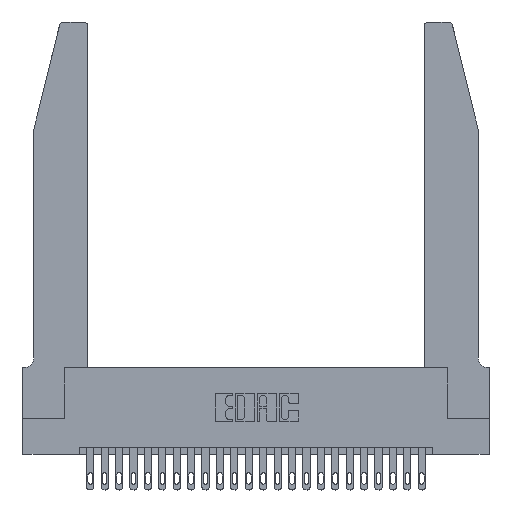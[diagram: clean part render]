
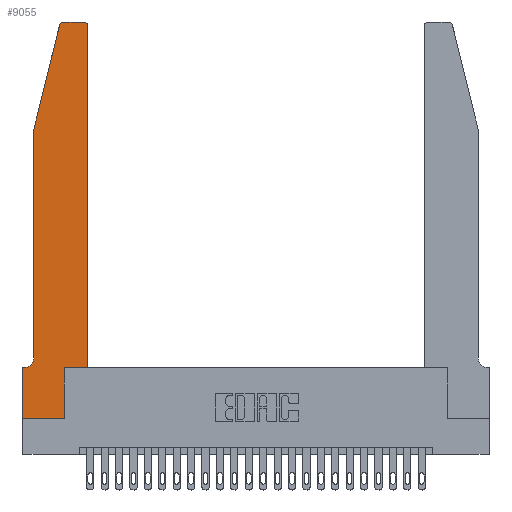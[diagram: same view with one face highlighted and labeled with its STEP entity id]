
A CAD part, top view. The second image highlights one B-rep face of the part: STEP entity #9055.
In plain terms, the highlighted planar face has unit normal (0, 0, 1).
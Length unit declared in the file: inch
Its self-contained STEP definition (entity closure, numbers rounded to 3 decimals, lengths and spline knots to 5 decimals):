
#1012 = VERTEX_POINT ( 'NONE', #17321 ) ;
#1343 = CARTESIAN_POINT ( 'NONE',  ( 0., 0., 0.37 ) ) ;
#1408 = DIRECTION ( 'NONE',  ( 0., 1., 0. ) ) ;
#1774 = ORIENTED_EDGE ( 'NONE', *, *, #21455, .T. ) ;
#2021 = VECTOR ( 'NONE', #23452, 39.37008 ) ;
#2440 = DIRECTION ( 'NONE',  ( -1., 0., 0. ) ) ;
#2599 = EDGE_CURVE ( 'NONE', #18158, #19687, #8711, .T. ) ;
#2645 = DIRECTION ( 'NONE',  ( 0., 0., 1. ) ) ;
#3170 = EDGE_CURVE ( 'NONE', #3212, #18158, #3987, .T. ) ;
#3212 = VERTEX_POINT ( 'NONE', #15938 ) ;
#3429 = LINE ( 'NONE', #4172, #18777 ) ;
#3468 = CARTESIAN_POINT ( 'NONE',  ( 0., 0., 0.37 ) ) ;
#3589 = LINE ( 'NONE', #13420, #18945 ) ;
#3613 = DIRECTION ( 'NONE',  ( 1., 0., 0. ) ) ;
#3987 = CIRCLE ( 'NONE', #25362, 0.03 ) ;
#4172 = CARTESIAN_POINT ( 'NONE',  ( 0.0755, 2., 0.37 ) ) ;
#4646 = VERTEX_POINT ( 'NONE', #13422 ) ;
#5094 = DIRECTION ( 'NONE',  ( 1., 0., 0. ) ) ;
#5379 = PLANE ( 'NONE',  #23579 ) ;
#6235 = CARTESIAN_POINT ( 'NONE',  ( 0.0755, 0.42, 0.37 ) ) ;
#7421 = EDGE_LOOP ( 'NONE', ( #23063, #25042, #14015, #12575, #7862, #16063, #1774, #9304, #20568, #23384, #13926, #14810 ) ) ;
#7805 = CARTESIAN_POINT ( 'NONE',  ( 0., 0.35, 0.37 ) ) ;
#7862 = ORIENTED_EDGE ( 'NONE', *, *, #20264, .T. ) ;
#8271 = CARTESIAN_POINT ( 'NONE',  ( 0.284, 2.75, 0.37 ) ) ;
#8536 = CARTESIAN_POINT ( 'NONE',  ( 0.284, 2.72, 0.37 ) ) ;
#8590 = CIRCLE ( 'NONE', #21376, 0.07 ) ;
#8711 = LINE ( 'NONE', #22270, #19089 ) ;
#8973 = VERTEX_POINT ( 'NONE', #1343 ) ;
#8981 = CARTESIAN_POINT ( 'NONE',  ( 0.2865, 0.35, 0.37 ) ) ;
#9055 = ADVANCED_FACE ( 'NONE', ( #25310 ), #5379, .T. ) ;
#9200 = LINE ( 'NONE', #11161, #15193 ) ;
#9304 = ORIENTED_EDGE ( 'NONE', *, *, #12291, .T. ) ;
#10670 = VECTOR ( 'NONE', #2440, 39.37008 ) ;
#11161 = CARTESIAN_POINT ( 'NONE',  ( 0., 0., 0.37 ) ) ;
#11275 = CIRCLE ( 'NONE', #17586, 0.03 ) ;
#11590 = VECTOR ( 'NONE', #5094, 39.37008 ) ;
#11944 = VERTEX_POINT ( 'NONE', #13131 ) ;
#12291 = EDGE_CURVE ( 'NONE', #8973, #13692, #16488, .T. ) ;
#12392 = DIRECTION ( 'NONE',  ( 1., 0., 0. ) ) ;
#12575 = ORIENTED_EDGE ( 'NONE', *, *, #21598, .T. ) ;
#13131 = CARTESIAN_POINT ( 'NONE',  ( 0.0755, 2., 0.37 ) ) ;
#13197 = CARTESIAN_POINT ( 'NONE',  ( 0.0055, 0.42, 0.37 ) ) ;
#13231 = VERTEX_POINT ( 'NONE', #8981 ) ;
#13420 = CARTESIAN_POINT ( 'NONE',  ( 0.0755, 2., 0.37 ) ) ;
#13422 = CARTESIAN_POINT ( 'NONE',  ( 0.0055, 0.35, 0.37 ) ) ;
#13692 = VERTEX_POINT ( 'NONE', #22928 ) ;
#13926 = ORIENTED_EDGE ( 'NONE', *, *, #18856, .T. ) ;
#14015 = ORIENTED_EDGE ( 'NONE', *, *, #17747, .T. ) ;
#14810 = ORIENTED_EDGE ( 'NONE', *, *, #3170, .T. ) ;
#15193 = VECTOR ( 'NONE', #19287, 39.37008 ) ;
#15235 = VECTOR ( 'NONE', #19707, 39.37008 ) ;
#15590 = LINE ( 'NONE', #16941, #23120 ) ;
#15938 = CARTESIAN_POINT ( 'NONE',  ( 0.4505, 2.72, 0.37 ) ) ;
#16063 = ORIENTED_EDGE ( 'NONE', *, *, #25273, .T. ) ;
#16488 = LINE ( 'NONE', #3468, #15235 ) ;
#16679 = VERTEX_POINT ( 'NONE', #6235 ) ;
#16941 = CARTESIAN_POINT ( 'NONE',  ( 0.4505, 0.35, 0.37 ) ) ;
#17083 = CARTESIAN_POINT ( 'NONE',  ( 0.4505, 0.35, 0.37 ) ) ;
#17321 = CARTESIAN_POINT ( 'NONE',  ( 0., 0.35, 0.37 ) ) ;
#17451 = DIRECTION ( 'NONE',  ( 0., -1., 0. ) ) ;
#17586 = AXIS2_PLACEMENT_3D ( 'NONE', #8536, #20426, #12392 ) ;
#17747 = EDGE_CURVE ( 'NONE', #20591, #11944, #3429, .T. ) ;
#17878 = LINE ( 'NONE', #20350, #10670 ) ;
#18158 = VERTEX_POINT ( 'NONE', #22478 ) ;
#18777 = VECTOR ( 'NONE', #22102, 39.37008 ) ;
#18826 = CARTESIAN_POINT ( 'NONE',  ( 0.4205, 2.72, 0.37 ) ) ;
#18856 = EDGE_CURVE ( 'NONE', #24229, #3212, #15590, .T. ) ;
#18945 = VECTOR ( 'NONE', #17451, 39.37008 ) ;
#19089 = VECTOR ( 'NONE', #22540, 39.37008 ) ;
#19287 = DIRECTION ( 'NONE',  ( 0., -1., 0. ) ) ;
#19687 = VERTEX_POINT ( 'NONE', #8271 ) ;
#19707 = DIRECTION ( 'NONE',  ( 1., 0., 0. ) ) ;
#19938 = DIRECTION ( 'NONE',  ( 0., 0., 1. ) ) ;
#20264 = EDGE_CURVE ( 'NONE', #16679, #4646, #8590, .T. ) ;
#20350 = CARTESIAN_POINT ( 'NONE',  ( 0.0755, 0.35, 0.37 ) ) ;
#20426 = DIRECTION ( 'NONE',  ( 0., 0., 1. ) ) ;
#20568 = ORIENTED_EDGE ( 'NONE', *, *, #20907, .T. ) ;
#20591 = VERTEX_POINT ( 'NONE', #23006 ) ;
#20907 = EDGE_CURVE ( 'NONE', #13692, #13231, #23937, .T. ) ;
#21232 = DIRECTION ( 'NONE',  ( 0., 0., -1. ) ) ;
#21376 = AXIS2_PLACEMENT_3D ( 'NONE', #13197, #21232, #22002 ) ;
#21455 = EDGE_CURVE ( 'NONE', #1012, #8973, #9200, .T. ) ;
#21598 = EDGE_CURVE ( 'NONE', #11944, #16679, #3589, .T. ) ;
#22002 = DIRECTION ( 'NONE',  ( -1., 0., 0. ) ) ;
#22102 = DIRECTION ( 'NONE',  ( -0.239, -0.971, 0. ) ) ;
#22270 = CARTESIAN_POINT ( 'NONE',  ( 0.2605, 2.75, 0.37 ) ) ;
#22478 = CARTESIAN_POINT ( 'NONE',  ( 0.4205, 2.75, 0.37 ) ) ;
#22540 = DIRECTION ( 'NONE',  ( -1., 0., 0. ) ) ;
#22928 = CARTESIAN_POINT ( 'NONE',  ( 0.2865, 0., 0.37 ) ) ;
#23006 = CARTESIAN_POINT ( 'NONE',  ( 0.25487, 2.72718, 0.37 ) ) ;
#23063 = ORIENTED_EDGE ( 'NONE', *, *, #2599, .T. ) ;
#23120 = VECTOR ( 'NONE', #1408, 39.37008 ) ;
#23293 = CARTESIAN_POINT ( 'NONE',  ( 0.2865, 0.35, 0.37 ) ) ;
#23384 = ORIENTED_EDGE ( 'NONE', *, *, #25652, .T. ) ;
#23452 = DIRECTION ( 'NONE',  ( 0., 1., 0. ) ) ;
#23579 = AXIS2_PLACEMENT_3D ( 'NONE', #7805, #19938, #3613 ) ;
#23937 = LINE ( 'NONE', #23293, #2021 ) ;
#24229 = VERTEX_POINT ( 'NONE', #24933 ) ;
#24933 = CARTESIAN_POINT ( 'NONE',  ( 0.4505, 0.35, 0.37 ) ) ;
#24968 = DIRECTION ( 'NONE',  ( 1., 0., 0. ) ) ;
#25042 = ORIENTED_EDGE ( 'NONE', *, *, #25912, .T. ) ;
#25105 = LINE ( 'NONE', #17083, #11590 ) ;
#25273 = EDGE_CURVE ( 'NONE', #4646, #1012, #17878, .T. ) ;
#25310 = FACE_OUTER_BOUND ( 'NONE', #7421, .T. ) ;
#25362 = AXIS2_PLACEMENT_3D ( 'NONE', #18826, #2645, #24968 ) ;
#25652 = EDGE_CURVE ( 'NONE', #13231, #24229, #25105, .T. ) ;
#25912 = EDGE_CURVE ( 'NONE', #19687, #20591, #11275, .T. ) ;
